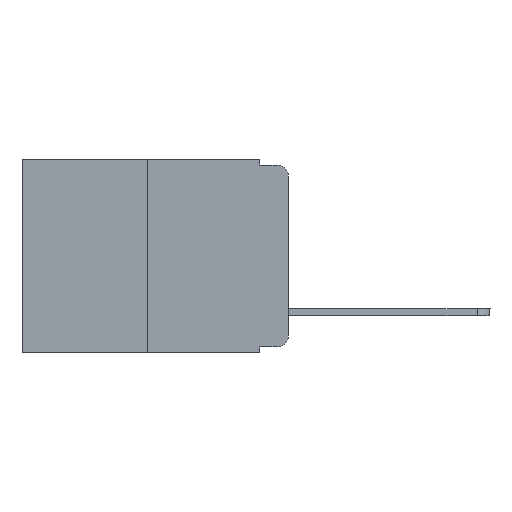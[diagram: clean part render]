
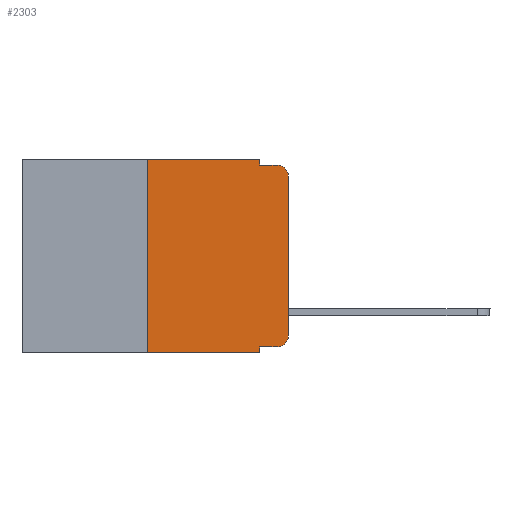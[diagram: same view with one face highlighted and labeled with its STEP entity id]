
A CAD part, left-side view. The second image highlights one B-rep face of the part: STEP entity #2303.
In plain terms, the highlighted planar face has unit normal (-1, 0, 0).
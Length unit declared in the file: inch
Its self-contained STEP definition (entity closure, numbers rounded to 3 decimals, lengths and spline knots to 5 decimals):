
#181 = DIRECTION ( 'NONE',  ( 0., 0., -1. ) ) ;
#192 = CARTESIAN_POINT ( 'NONE',  ( 0., 0., -0.03 ) ) ;
#1094 = VERTEX_POINT ( 'NONE', #5594 ) ;
#1532 = EDGE_CURVE ( 'NONE', #20082, #5648, #21634, .T. ) ;
#1638 = CARTESIAN_POINT ( 'NONE',  ( 0., 0.473, 0. ) ) ;
#1694 = EDGE_CURVE ( 'NONE', #1094, #2985, #16936, .T. ) ;
#1852 = CARTESIAN_POINT ( 'NONE',  ( 0., 0.02, -0.313 ) ) ;
#1924 = DIRECTION ( 'NONE',  ( -1., 0., 0. ) ) ;
#2191 = ORIENTED_EDGE ( 'NONE', *, *, #5102, .F. ) ;
#2303 = ADVANCED_FACE ( 'NONE', ( #2973 ), #18618, .F. ) ;
#2578 = DIRECTION ( 'NONE',  ( -1., 0., 0. ) ) ;
#2686 = LINE ( 'NONE', #18377, #11914 ) ;
#2973 = FACE_OUTER_BOUND ( 'NONE', #6034, .T. ) ;
#2985 = VERTEX_POINT ( 'NONE', #3657 ) ;
#3150 = DIRECTION ( 'NONE',  ( 0., -1., 0. ) ) ;
#3206 = CARTESIAN_POINT ( 'NONE',  ( 0., 0.25, 0. ) ) ;
#3610 = DIRECTION ( 'NONE',  ( 1., 0., 0. ) ) ;
#3657 = CARTESIAN_POINT ( 'NONE',  ( 0., 0.051, -0.01 ) ) ;
#3798 = LINE ( 'NONE', #13208, #17188 ) ;
#3830 = VERTEX_POINT ( 'NONE', #4127 ) ;
#4127 = CARTESIAN_POINT ( 'NONE',  ( 0., 0.25, 0. ) ) ;
#4948 = CARTESIAN_POINT ( 'NONE',  ( 0., 0.051, -0.333 ) ) ;
#5102 = EDGE_CURVE ( 'NONE', #20082, #20218, #2686, .T. ) ;
#5415 = DIRECTION ( 'NONE',  ( 0., 0., 1. ) ) ;
#5594 = CARTESIAN_POINT ( 'NONE',  ( 0., 0.051, 0. ) ) ;
#5648 = VERTEX_POINT ( 'NONE', #15639 ) ;
#5685 = ORIENTED_EDGE ( 'NONE', *, *, #1694, .F. ) ;
#6034 = EDGE_LOOP ( 'NONE', ( #8133, #18145, #11493, #5685, #7604, #19577, #20355, #2191, #14361, #20746 ) ) ;
#6462 = CARTESIAN_POINT ( 'NONE',  ( 0., 0.02, -0.01 ) ) ;
#6482 = EDGE_CURVE ( 'NONE', #3830, #1094, #14680, .T. ) ;
#6831 = VECTOR ( 'NONE', #12838, 39.37008 ) ;
#7137 = AXIS2_PLACEMENT_3D ( 'NONE', #1638, #3610, #181 ) ;
#7604 = ORIENTED_EDGE ( 'NONE', *, *, #6482, .F. ) ;
#8133 = ORIENTED_EDGE ( 'NONE', *, *, #10282, .T. ) ;
#8322 = DIRECTION ( 'NONE',  ( 0., 0., -1. ) ) ;
#8356 = DIRECTION ( 'NONE',  ( 0., -1., 0. ) ) ;
#8937 = CIRCLE ( 'NONE', #15218, 0.02 ) ;
#9537 = VERTEX_POINT ( 'NONE', #192 ) ;
#10028 = CARTESIAN_POINT ( 'NONE',  ( 0., 0., 0. ) ) ;
#10270 = AXIS2_PLACEMENT_3D ( 'NONE', #11957, #2578, #21681 ) ;
#10282 = EDGE_CURVE ( 'NONE', #19359, #9537, #17657, .T. ) ;
#10816 = VERTEX_POINT ( 'NONE', #6462 ) ;
#11309 = CARTESIAN_POINT ( 'NONE',  ( 0., 0.473, 0. ) ) ;
#11493 = ORIENTED_EDGE ( 'NONE', *, *, #21307, .F. ) ;
#11704 = DIRECTION ( 'NONE',  ( 0., -1., 0. ) ) ;
#11911 = CARTESIAN_POINT ( 'NONE',  ( 0., 0.051, -0.343 ) ) ;
#11914 = VECTOR ( 'NONE', #8322, 39.37008 ) ;
#11957 = CARTESIAN_POINT ( 'NONE',  ( 0., 0.02, -0.03 ) ) ;
#12057 = CARTESIAN_POINT ( 'NONE',  ( 0., 0.25, -0.343 ) ) ;
#12126 = DIRECTION ( 'NONE',  ( 0., 0., -1. ) ) ;
#12343 = VERTEX_POINT ( 'NONE', #12057 ) ;
#12838 = DIRECTION ( 'NONE',  ( 0., -1., 0. ) ) ;
#13075 = CARTESIAN_POINT ( 'NONE',  ( 0., 0.051, -0.333 ) ) ;
#13208 = CARTESIAN_POINT ( 'NONE',  ( 0., 0.051, -0.01 ) ) ;
#13295 = EDGE_CURVE ( 'NONE', #12343, #3830, #15459, .T. ) ;
#13743 = VECTOR ( 'NONE', #5415, 39.37008 ) ;
#14045 = EDGE_CURVE ( 'NONE', #9537, #10816, #20140, .T. ) ;
#14361 = ORIENTED_EDGE ( 'NONE', *, *, #1532, .T. ) ;
#14680 = LINE ( 'NONE', #11309, #6831 ) ;
#15218 = AXIS2_PLACEMENT_3D ( 'NONE', #1852, #1924, #12126 ) ;
#15459 = LINE ( 'NONE', #3206, #17296 ) ;
#15558 = CARTESIAN_POINT ( 'NONE',  ( 0., 0., -0.313 ) ) ;
#15639 = CARTESIAN_POINT ( 'NONE',  ( 0., 0.02, -0.333 ) ) ;
#16348 = VECTOR ( 'NONE', #8356, 39.37008 ) ;
#16558 = EDGE_CURVE ( 'NONE', #5648, #19359, #8937, .T. ) ;
#16936 = LINE ( 'NONE', #19904, #21378 ) ;
#17188 = VECTOR ( 'NONE', #3150, 39.37008 ) ;
#17296 = VECTOR ( 'NONE', #18305, 39.37008 ) ;
#17657 = LINE ( 'NONE', #10028, #13743 ) ;
#17693 = VECTOR ( 'NONE', #11704, 39.37008 ) ;
#17924 = EDGE_CURVE ( 'NONE', #12343, #20218, #18697, .T. ) ;
#18145 = ORIENTED_EDGE ( 'NONE', *, *, #14045, .T. ) ;
#18230 = DIRECTION ( 'NONE',  ( 0., 0., -1. ) ) ;
#18305 = DIRECTION ( 'NONE',  ( 0., 0., 1. ) ) ;
#18377 = CARTESIAN_POINT ( 'NONE',  ( 0., 0.051, 0. ) ) ;
#18618 = PLANE ( 'NONE',  #7137 ) ;
#18697 = LINE ( 'NONE', #19958, #16348 ) ;
#19359 = VERTEX_POINT ( 'NONE', #15558 ) ;
#19577 = ORIENTED_EDGE ( 'NONE', *, *, #13295, .F. ) ;
#19904 = CARTESIAN_POINT ( 'NONE',  ( 0., 0.051, 0. ) ) ;
#19958 = CARTESIAN_POINT ( 'NONE',  ( 0., 0.473, -0.343 ) ) ;
#20082 = VERTEX_POINT ( 'NONE', #13075 ) ;
#20140 = CIRCLE ( 'NONE', #10270, 0.02 ) ;
#20218 = VERTEX_POINT ( 'NONE', #11911 ) ;
#20355 = ORIENTED_EDGE ( 'NONE', *, *, #17924, .T. ) ;
#20746 = ORIENTED_EDGE ( 'NONE', *, *, #16558, .T. ) ;
#21307 = EDGE_CURVE ( 'NONE', #2985, #10816, #3798, .T. ) ;
#21378 = VECTOR ( 'NONE', #18230, 39.37008 ) ;
#21634 = LINE ( 'NONE', #4948, #17693 ) ;
#21681 = DIRECTION ( 'NONE',  ( 0., 0., -1. ) ) ;
